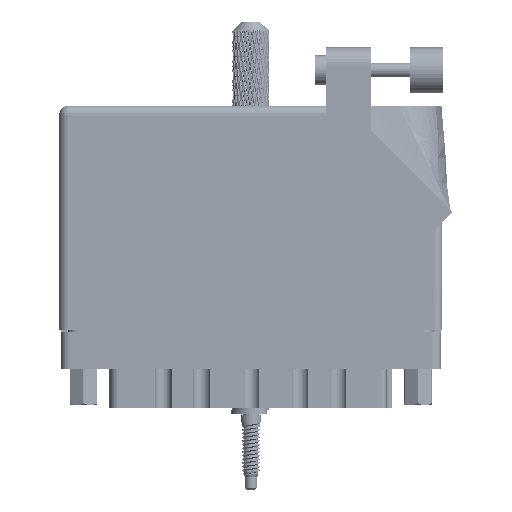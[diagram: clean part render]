
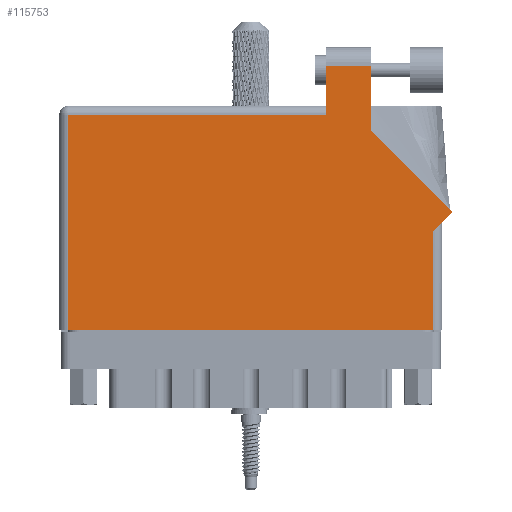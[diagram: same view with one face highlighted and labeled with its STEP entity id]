
A CAD part, front view. The second image highlights one B-rep face of the part: STEP entity #115753.
In plain terms, the highlighted face is planar.
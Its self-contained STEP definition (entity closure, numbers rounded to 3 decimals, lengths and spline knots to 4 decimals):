
#965 = EDGE_CURVE ( 'NONE', #73742, #40925, #55971, .T. ) ;
#3766 = EDGE_CURVE ( 'NONE', #47508, #12325, #107926, .T. ) ;
#4456 = CARTESIAN_POINT ( 'NONE',  ( 0., 1.468, 0. ) ) ;
#6753 = VERTEX_POINT ( 'NONE', #121599 ) ;
#7644 = ORIENTED_EDGE ( 'NONE', *, *, #40163, .T. ) ;
#8697 = FACE_OUTER_BOUND ( 'NONE', #126146, .T. ) ;
#10144 = EDGE_CURVE ( 'NONE', #78526, #6753, #106779, .T. ) ;
#11405 = DIRECTION ( 'NONE',  ( 0., 1., 0. ) ) ;
#11711 = CARTESIAN_POINT ( 'NONE',  ( 0.062, 0., 0. ) ) ;
#12325 = VERTEX_POINT ( 'NONE', #56261 ) ;
#12992 = ORIENTED_EDGE ( 'NONE', *, *, #31383, .T. ) ;
#13430 = EDGE_CURVE ( 'NONE', #92045, #78526, #70598, .T. ) ;
#15955 = VERTEX_POINT ( 'NONE', #52094 ) ;
#16717 = VECTOR ( 'NONE', #123235, 39.3701 ) ;
#16798 = CARTESIAN_POINT ( 'NONE',  ( 1.819, 1.805, 0. ) ) ;
#18396 = VECTOR ( 'NONE', #88943, 39.3701 ) ;
#20303 = DIRECTION ( 'NONE',  ( -1., 0., 0. ) ) ;
#22388 = ORIENTED_EDGE ( 'NONE', *, *, #965, .T. ) ;
#24080 = ORIENTED_EDGE ( 'NONE', *, *, #10144, .T. ) ;
#26357 = VECTOR ( 'NONE', #65388, 39.3701 ) ;
#31383 = EDGE_CURVE ( 'NONE', #40925, #47508, #101249, .T. ) ;
#32187 = VECTOR ( 'NONE', #70870, 39.3701 ) ;
#32923 = CARTESIAN_POINT ( 'NONE',  ( 0.062, 1.468, 0. ) ) ;
#34094 = CARTESIAN_POINT ( 'NONE',  ( 1.819, 1.468, 0. ) ) ;
#36927 = ORIENTED_EDGE ( 'NONE', *, *, #91268, .T. ) ;
#39627 = DIRECTION ( 'NONE',  ( 0., 0., -1. ) ) ;
#40163 = EDGE_CURVE ( 'NONE', #6753, #73742, #67869, .T. ) ;
#40925 = VERTEX_POINT ( 'NONE', #34094 ) ;
#44662 = CARTESIAN_POINT ( 'NONE',  ( 2.6827, 0.8077, 0. ) ) ;
#45085 = CARTESIAN_POINT ( 'NONE',  ( 2.55, 0.737, 0. ) ) ;
#47508 = VERTEX_POINT ( 'NONE', #32923 ) ;
#51761 = CARTESIAN_POINT ( 'NONE',  ( 2.55, 0., 0. ) ) ;
#52094 = CARTESIAN_POINT ( 'NONE',  ( 2.55, 0.675, 0. ) ) ;
#52581 = LINE ( 'NONE', #45085, #26357 ) ;
#55009 = VECTOR ( 'NONE', #73206, 39.3701 ) ;
#55971 = LINE ( 'NONE', #107976, #99224 ) ;
#56039 = ORIENTED_EDGE ( 'NONE', *, *, #13430, .T. ) ;
#56261 = CARTESIAN_POINT ( 'NONE',  ( 0.062, 0., 0. ) ) ;
#59150 = DIRECTION ( 'NONE',  ( 0., -1., 0. ) ) ;
#62115 = ORIENTED_EDGE ( 'NONE', *, *, #78626, .T. ) ;
#62335 = CARTESIAN_POINT ( 'NONE',  ( 2.6827, 0.8077, 0. ) ) ;
#62408 = CARTESIAN_POINT ( 'NONE',  ( 2.612, 0.737, 0. ) ) ;
#64533 = DIRECTION ( 'NONE',  ( -1., 0., 0. ) ) ;
#65388 = DIRECTION ( 'NONE',  ( 0., 1., 0. ) ) ;
#67869 = LINE ( 'NONE', #119199, #125088 ) ;
#70598 = LINE ( 'NONE', #62335, #16717 ) ;
#70870 = DIRECTION ( 'NONE',  ( 0., -1., 0. ) ) ;
#73206 = DIRECTION ( 'NONE',  ( 0.707, 0.707, 0. ) ) ;
#73742 = VERTEX_POINT ( 'NONE', #16798 ) ;
#78073 = VECTOR ( 'NONE', #122384, 39.3701 ) ;
#78526 = VERTEX_POINT ( 'NONE', #110753 ) ;
#78626 = EDGE_CURVE ( 'NONE', #119681, #15955, #52581, .T. ) ;
#88479 = PLANE ( 'NONE',  #108899 ) ;
#88901 = CARTESIAN_POINT ( 'NONE',  ( 0., 1.53, 0. ) ) ;
#88943 = DIRECTION ( 'NONE',  ( 1., 0., 0. ) ) ;
#91268 = EDGE_CURVE ( 'NONE', #15955, #92045, #101386, .T. ) ;
#92045 = VERTEX_POINT ( 'NONE', #44662 ) ;
#92576 = CARTESIAN_POINT ( 'NONE',  ( 2.126, 1.3644, 0. ) ) ;
#99224 = VECTOR ( 'NONE', #59150, 39.3701 ) ;
#101249 = LINE ( 'NONE', #4456, #78073 ) ;
#101386 = LINE ( 'NONE', #62408, #55009 ) ;
#103644 = ORIENTED_EDGE ( 'NONE', *, *, #113578, .T. ) ;
#106779 = LINE ( 'NONE', #92576, #111337 ) ;
#107926 = LINE ( 'NONE', #11711, #32187 ) ;
#107976 = CARTESIAN_POINT ( 'NONE',  ( 1.819, 1.53, 0. ) ) ;
#108899 = AXIS2_PLACEMENT_3D ( 'NONE', #88901, #39627, #20303 ) ;
#110753 = CARTESIAN_POINT ( 'NONE',  ( 2.126, 1.3644, 0. ) ) ;
#111337 = VECTOR ( 'NONE', #11405, 39.3701 ) ;
#113578 = EDGE_CURVE ( 'NONE', #12325, #119681, #128071, .T. ) ;
#115753 = ADVANCED_FACE ( 'NONE', ( #8697 ), #88479, .F. ) ;
#119066 = ORIENTED_EDGE ( 'NONE', *, *, #3766, .T. ) ;
#119199 = CARTESIAN_POINT ( 'NONE',  ( 1.819, 1.805, 0. ) ) ;
#119630 = CARTESIAN_POINT ( 'NONE',  ( 0., 0., 0. ) ) ;
#119681 = VERTEX_POINT ( 'NONE', #51761 ) ;
#121599 = CARTESIAN_POINT ( 'NONE',  ( 2.126, 1.805, 0. ) ) ;
#122384 = DIRECTION ( 'NONE',  ( -1., 0., 0. ) ) ;
#123235 = DIRECTION ( 'NONE',  ( -0.707, 0.707, 0. ) ) ;
#125088 = VECTOR ( 'NONE', #64533, 39.3701 ) ;
#126146 = EDGE_LOOP ( 'NONE', ( #24080, #7644, #22388, #12992, #119066, #103644, #62115, #36927, #56039 ) ) ;
#128071 = LINE ( 'NONE', #119630, #18396 ) ;
